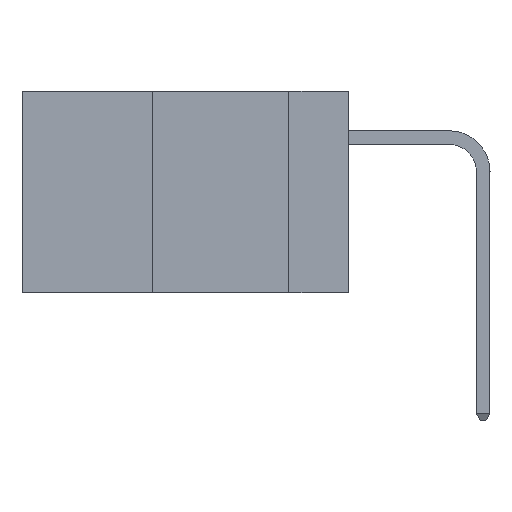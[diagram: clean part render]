
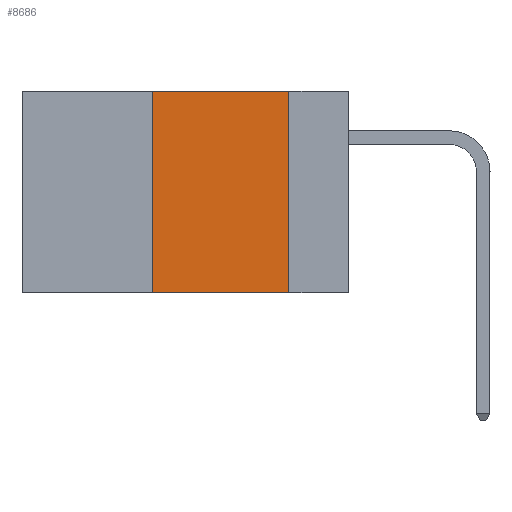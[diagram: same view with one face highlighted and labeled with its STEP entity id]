
A CAD part, left-side view. The second image highlights one B-rep face of the part: STEP entity #8686.
In plain terms, the highlighted planar face has unit normal (-1, 0, 0).
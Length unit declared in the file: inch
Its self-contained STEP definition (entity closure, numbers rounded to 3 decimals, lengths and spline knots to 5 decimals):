
#1217 = ORIENTED_EDGE ( 'NONE', *, *, #18774, .F. ) ;
#1532 = PLANE ( 'NONE',  #20940 ) ;
#2063 = ORIENTED_EDGE ( 'NONE', *, *, #11272, .F. ) ;
#3971 = DIRECTION ( 'NONE',  ( 0., 0., -1. ) ) ;
#4592 = VECTOR ( 'NONE', #20488, 39.37008 ) ;
#4628 = CARTESIAN_POINT ( 'NONE',  ( 0., 0.6, 0. ) ) ;
#5192 = LINE ( 'NONE', #15846, #18644 ) ;
#6060 = VECTOR ( 'NONE', #3971, 39.37008 ) ;
#6189 = DIRECTION ( 'NONE',  ( 0., 0., -1. ) ) ;
#8269 = VERTEX_POINT ( 'NONE', #18182 ) ;
#8686 = ADVANCED_FACE ( 'NONE', ( #13805 ), #1532, .F. ) ;
#9526 = EDGE_CURVE ( 'NONE', #11930, #8269, #5192, .T. ) ;
#10373 = CARTESIAN_POINT ( 'NONE',  ( 0., 0.6, 0. ) ) ;
#10968 = CARTESIAN_POINT ( 'NONE',  ( 0., 0.36, 0. ) ) ;
#11115 = DIRECTION ( 'NONE',  ( 0., -1., 0. ) ) ;
#11272 = EDGE_CURVE ( 'NONE', #27000, #8269, #12068, .T. ) ;
#11930 = VERTEX_POINT ( 'NONE', #24384 ) ;
#12068 = LINE ( 'NONE', #17815, #6060 ) ;
#12532 = ORIENTED_EDGE ( 'NONE', *, *, #13021, .F. ) ;
#13021 = EDGE_CURVE ( 'NONE', #11930, #18308, #28999, .T. ) ;
#13805 = FACE_OUTER_BOUND ( 'NONE', #21929, .T. ) ;
#15107 = DIRECTION ( 'NONE',  ( 0., 0., 1. ) ) ;
#15846 = CARTESIAN_POINT ( 'NONE',  ( 0., 0.6, -0.37 ) ) ;
#17815 = CARTESIAN_POINT ( 'NONE',  ( 0., 0.11, 0. ) ) ;
#18182 = CARTESIAN_POINT ( 'NONE',  ( 0., 0.11, -0.37 ) ) ;
#18308 = VERTEX_POINT ( 'NONE', #25954 ) ;
#18644 = VECTOR ( 'NONE', #11115, 39.37008 ) ;
#18774 = EDGE_CURVE ( 'NONE', #18308, #27000, #26232, .T. ) ;
#19080 = ORIENTED_EDGE ( 'NONE', *, *, #9526, .T. ) ;
#20488 = DIRECTION ( 'NONE',  ( 0., -1., 0. ) ) ;
#20940 = AXIS2_PLACEMENT_3D ( 'NONE', #10373, #21862, #6189 ) ;
#21862 = DIRECTION ( 'NONE',  ( 1., 0., 0. ) ) ;
#21929 = EDGE_LOOP ( 'NONE', ( #2063, #1217, #12532, #19080 ) ) ;
#22634 = CARTESIAN_POINT ( 'NONE',  ( 0., 0.11, 0. ) ) ;
#23713 = VECTOR ( 'NONE', #15107, 39.37008 ) ;
#24384 = CARTESIAN_POINT ( 'NONE',  ( 0., 0.36, -0.37 ) ) ;
#25954 = CARTESIAN_POINT ( 'NONE',  ( 0., 0.36, 0. ) ) ;
#26232 = LINE ( 'NONE', #4628, #4592 ) ;
#27000 = VERTEX_POINT ( 'NONE', #22634 ) ;
#28999 = LINE ( 'NONE', #10968, #23713 ) ;
